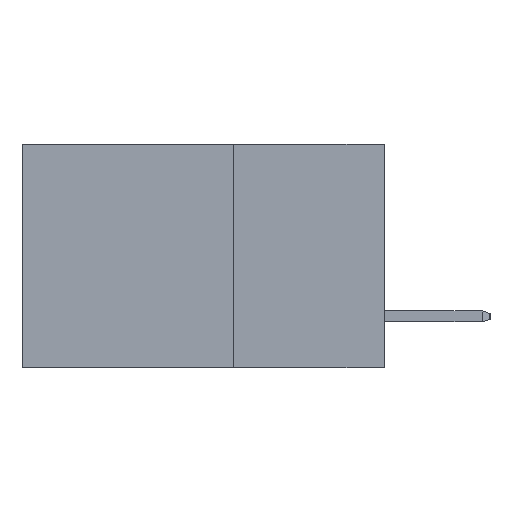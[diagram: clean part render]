
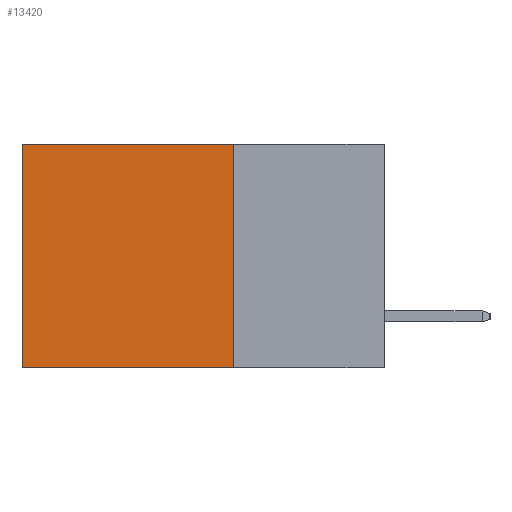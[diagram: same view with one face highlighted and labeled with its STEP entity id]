
A CAD part, left-side view. The second image highlights one B-rep face of the part: STEP entity #13420.
In plain terms, the highlighted planar face has unit normal (-1, 0, 0).
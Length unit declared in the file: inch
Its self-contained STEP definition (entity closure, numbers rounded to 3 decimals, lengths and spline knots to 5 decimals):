
#4 = CARTESIAN_POINT ( 'NONE',  ( 0.298, 0.6, 0. ) ) ;
#72 = LINE ( 'NONE', #11820, #9581 ) ;
#124 = CARTESIAN_POINT ( 'NONE',  ( 0.298, 0.25, 0. ) ) ;
#904 = VECTOR ( 'NONE', #12757, 39.37008 ) ;
#1533 = VECTOR ( 'NONE', #15612, 39.37008 ) ;
#2172 = VECTOR ( 'NONE', #14261, 39.37008 ) ;
#2496 = CARTESIAN_POINT ( 'NONE',  ( 0.298, 0.6, 0. ) ) ;
#2762 = DIRECTION ( 'NONE',  ( 1., 0., 0. ) ) ;
#2871 = EDGE_LOOP ( 'NONE', ( #3394, #14467, #11540, #12751 ) ) ;
#3394 = ORIENTED_EDGE ( 'NONE', *, *, #16289, .T. ) ;
#3720 = CARTESIAN_POINT ( 'NONE',  ( 0.298, 0.25, 0. ) ) ;
#3997 = EDGE_CURVE ( 'NONE', #13284, #10493, #72, .T. ) ;
#4152 = CARTESIAN_POINT ( 'NONE',  ( 0.298, 0.25, 0. ) ) ;
#4175 = CARTESIAN_POINT ( 'NONE',  ( 0.298, 0.6, -0.37 ) ) ;
#4333 = LINE ( 'NONE', #2496, #904 ) ;
#5142 = AXIS2_PLACEMENT_3D ( 'NONE', #124, #2762, #11737 ) ;
#6611 = CARTESIAN_POINT ( 'NONE',  ( 0.298, 0.25, -0.37 ) ) ;
#7661 = FACE_OUTER_BOUND ( 'NONE', #2871, .T. ) ;
#8999 = EDGE_CURVE ( 'NONE', #10493, #10323, #15690, .T. ) ;
#9581 = VECTOR ( 'NONE', #13480, 39.37008 ) ;
#10323 = VERTEX_POINT ( 'NONE', #4175 ) ;
#10493 = VERTEX_POINT ( 'NONE', #15897 ) ;
#11540 = ORIENTED_EDGE ( 'NONE', *, *, #3997, .F. ) ;
#11580 = VERTEX_POINT ( 'NONE', #4 ) ;
#11737 = DIRECTION ( 'NONE',  ( 0., 0., -1. ) ) ;
#11775 = LINE ( 'NONE', #4152, #1533 ) ;
#11820 = CARTESIAN_POINT ( 'NONE',  ( 0.298, 0.25, 0. ) ) ;
#12751 = ORIENTED_EDGE ( 'NONE', *, *, #16485, .T. ) ;
#12757 = DIRECTION ( 'NONE',  ( 0., 0., -1. ) ) ;
#12968 = PLANE ( 'NONE',  #5142 ) ;
#13284 = VERTEX_POINT ( 'NONE', #3720 ) ;
#13420 = ADVANCED_FACE ( 'NONE', ( #7661 ), #12968, .F. ) ;
#13480 = DIRECTION ( 'NONE',  ( 0., 0., -1. ) ) ;
#14261 = DIRECTION ( 'NONE',  ( 0., 1., 0. ) ) ;
#14467 = ORIENTED_EDGE ( 'NONE', *, *, #8999, .F. ) ;
#15612 = DIRECTION ( 'NONE',  ( 0., 1., 0. ) ) ;
#15690 = LINE ( 'NONE', #6611, #2172 ) ;
#15897 = CARTESIAN_POINT ( 'NONE',  ( 0.298, 0.25, -0.37 ) ) ;
#16289 = EDGE_CURVE ( 'NONE', #11580, #10323, #4333, .T. ) ;
#16485 = EDGE_CURVE ( 'NONE', #13284, #11580, #11775, .T. ) ;
